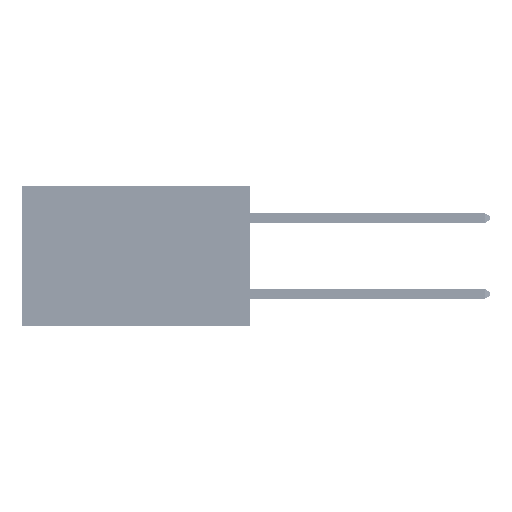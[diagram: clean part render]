
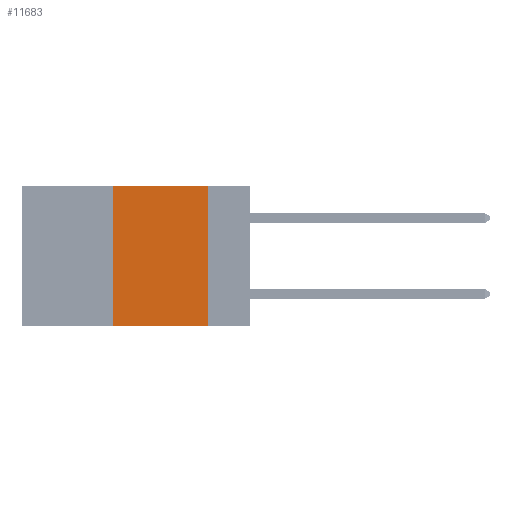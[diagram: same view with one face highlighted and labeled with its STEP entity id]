
A CAD part, left-side view. The second image highlights one B-rep face of the part: STEP entity #11683.
In plain terms, the highlighted planar face has unit normal (-1, 0, 0).
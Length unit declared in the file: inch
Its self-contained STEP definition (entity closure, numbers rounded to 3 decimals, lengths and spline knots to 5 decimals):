
#487 = AXIS2_PLACEMENT_3D ( 'NONE', #6935, #14438, #26671 ) ;
#2645 = ORIENTED_EDGE ( 'NONE', *, *, #30811, .T. ) ;
#2858 = DIRECTION ( 'NONE',  ( 0., 0., -1. ) ) ;
#4688 = CARTESIAN_POINT ( 'NONE',  ( 0., 0.36, 0. ) ) ;
#4833 = VECTOR ( 'NONE', #28616, 39.37008 ) ;
#5761 = VECTOR ( 'NONE', #12375, 39.37008 ) ;
#6141 = VECTOR ( 'NONE', #51498, 39.37008 ) ;
#6209 = CARTESIAN_POINT ( 'NONE',  ( 0., 0.6, 0. ) ) ;
#6214 = ORIENTED_EDGE ( 'NONE', *, *, #9583, .F. ) ;
#6935 = CARTESIAN_POINT ( 'NONE',  ( 0., 0.6, 0. ) ) ;
#9583 = EDGE_CURVE ( 'NONE', #13673, #24004, #22345, .T. ) ;
#11683 = ADVANCED_FACE ( 'NONE', ( #45608 ), #43152, .F. ) ;
#12375 = DIRECTION ( 'NONE',  ( 0., 0., 1. ) ) ;
#13673 = VERTEX_POINT ( 'NONE', #43957 ) ;
#14438 = DIRECTION ( 'NONE',  ( 1., 0., 0. ) ) ;
#16033 = CARTESIAN_POINT ( 'NONE',  ( 0., 0.36, 0. ) ) ;
#19526 = CARTESIAN_POINT ( 'NONE',  ( 0., 0.11, -0.37 ) ) ;
#20621 = ORIENTED_EDGE ( 'NONE', *, *, #48108, .F. ) ;
#22345 = LINE ( 'NONE', #4688, #5761 ) ;
#23506 = VERTEX_POINT ( 'NONE', #19526 ) ;
#24004 = VERTEX_POINT ( 'NONE', #16033 ) ;
#26671 = DIRECTION ( 'NONE',  ( 0., 0., -1. ) ) ;
#28267 = EDGE_LOOP ( 'NONE', ( #50277, #20621, #6214, #2645 ) ) ;
#28616 = DIRECTION ( 'NONE',  ( 0., -1., 0. ) ) ;
#30811 = EDGE_CURVE ( 'NONE', #13673, #23506, #48663, .T. ) ;
#31670 = CARTESIAN_POINT ( 'NONE',  ( 0., 0.6, -0.37 ) ) ;
#34171 = VECTOR ( 'NONE', #2858, 39.37008 ) ;
#35437 = LINE ( 'NONE', #6209, #6141 ) ;
#38301 = VERTEX_POINT ( 'NONE', #45907 ) ;
#43152 = PLANE ( 'NONE',  #487 ) ;
#43957 = CARTESIAN_POINT ( 'NONE',  ( 0., 0.36, -0.37 ) ) ;
#44911 = LINE ( 'NONE', #51549, #34171 ) ;
#45608 = FACE_OUTER_BOUND ( 'NONE', #28267, .T. ) ;
#45907 = CARTESIAN_POINT ( 'NONE',  ( 0., 0.11, 0. ) ) ;
#47978 = EDGE_CURVE ( 'NONE', #38301, #23506, #44911, .T. ) ;
#48108 = EDGE_CURVE ( 'NONE', #24004, #38301, #35437, .T. ) ;
#48663 = LINE ( 'NONE', #31670, #4833 ) ;
#50277 = ORIENTED_EDGE ( 'NONE', *, *, #47978, .F. ) ;
#51498 = DIRECTION ( 'NONE',  ( 0., -1., 0. ) ) ;
#51549 = CARTESIAN_POINT ( 'NONE',  ( 0., 0.11, 0. ) ) ;
